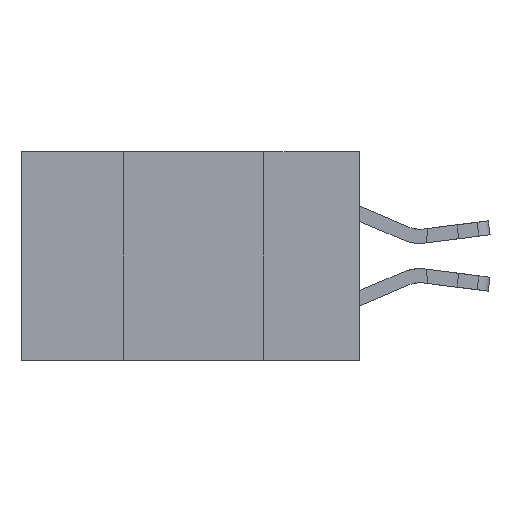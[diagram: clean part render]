
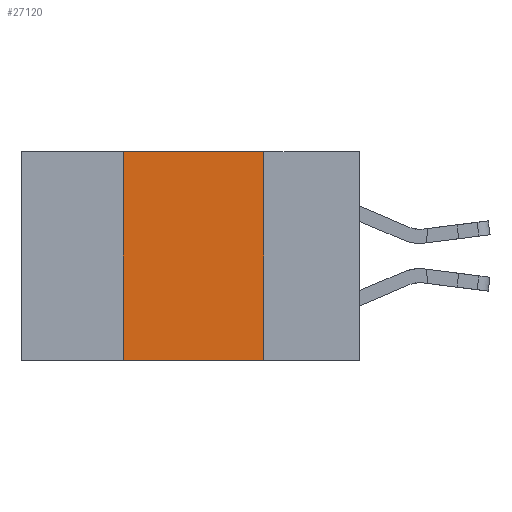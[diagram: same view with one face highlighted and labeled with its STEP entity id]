
A CAD part, left-side view. The second image highlights one B-rep face of the part: STEP entity #27120.
In plain terms, the highlighted planar face has unit normal (-1, 0, 0).
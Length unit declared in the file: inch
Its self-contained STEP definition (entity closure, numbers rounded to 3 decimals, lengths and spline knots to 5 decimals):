
#164 = CARTESIAN_POINT ( 'NONE',  ( 0., 0.6, 0. ) ) ;
#171 = EDGE_CURVE ( 'NONE', #13686, #13210, #23128, .T. ) ;
#1708 = CARTESIAN_POINT ( 'NONE',  ( 0., 0.42, 0. ) ) ;
#1950 = VECTOR ( 'NONE', #25663, 39.37008 ) ;
#2066 = CARTESIAN_POINT ( 'NONE',  ( 0., 0.17, 0. ) ) ;
#2390 = FACE_OUTER_BOUND ( 'NONE', #27719, .T. ) ;
#3191 = LINE ( 'NONE', #14904, #5204 ) ;
#3669 = ORIENTED_EDGE ( 'NONE', *, *, #11822, .F. ) ;
#5204 = VECTOR ( 'NONE', #23790, 39.37008 ) ;
#6777 = CARTESIAN_POINT ( 'NONE',  ( 0., 0.17, 0. ) ) ;
#8789 = DIRECTION ( 'NONE',  ( 0., 0., -1. ) ) ;
#9563 = CARTESIAN_POINT ( 'NONE',  ( 0., 0.17, -0.37 ) ) ;
#9866 = VERTEX_POINT ( 'NONE', #23893 ) ;
#11260 = LINE ( 'NONE', #2066, #17784 ) ;
#11659 = LINE ( 'NONE', #23503, #23177 ) ;
#11822 = EDGE_CURVE ( 'NONE', #13210, #20097, #11260, .T. ) ;
#13210 = VERTEX_POINT ( 'NONE', #6777 ) ;
#13564 = ORIENTED_EDGE ( 'NONE', *, *, #171, .F. ) ;
#13686 = VERTEX_POINT ( 'NONE', #1708 ) ;
#14452 = ORIENTED_EDGE ( 'NONE', *, *, #18312, .F. ) ;
#14904 = CARTESIAN_POINT ( 'NONE',  ( 0., 0.6, -0.37 ) ) ;
#15165 = AXIS2_PLACEMENT_3D ( 'NONE', #164, #18094, #8789 ) ;
#16682 = ORIENTED_EDGE ( 'NONE', *, *, #26409, .T. ) ;
#17784 = VECTOR ( 'NONE', #27270, 39.37008 ) ;
#18094 = DIRECTION ( 'NONE',  ( 1., 0., 0. ) ) ;
#18312 = EDGE_CURVE ( 'NONE', #9866, #13686, #11659, .T. ) ;
#20097 = VERTEX_POINT ( 'NONE', #9563 ) ;
#23128 = LINE ( 'NONE', #27611, #1950 ) ;
#23177 = VECTOR ( 'NONE', #23211, 39.37008 ) ;
#23211 = DIRECTION ( 'NONE',  ( 0., 0., 1. ) ) ;
#23503 = CARTESIAN_POINT ( 'NONE',  ( 0., 0.42, 0. ) ) ;
#23790 = DIRECTION ( 'NONE',  ( 0., -1., 0. ) ) ;
#23893 = CARTESIAN_POINT ( 'NONE',  ( 0., 0.42, -0.37 ) ) ;
#24627 = PLANE ( 'NONE',  #15165 ) ;
#25663 = DIRECTION ( 'NONE',  ( 0., -1., 0. ) ) ;
#26409 = EDGE_CURVE ( 'NONE', #9866, #20097, #3191, .T. ) ;
#27120 = ADVANCED_FACE ( 'NONE', ( #2390 ), #24627, .F. ) ;
#27270 = DIRECTION ( 'NONE',  ( 0., 0., -1. ) ) ;
#27611 = CARTESIAN_POINT ( 'NONE',  ( 0., 0.6, 0. ) ) ;
#27719 = EDGE_LOOP ( 'NONE', ( #3669, #13564, #14452, #16682 ) ) ;
